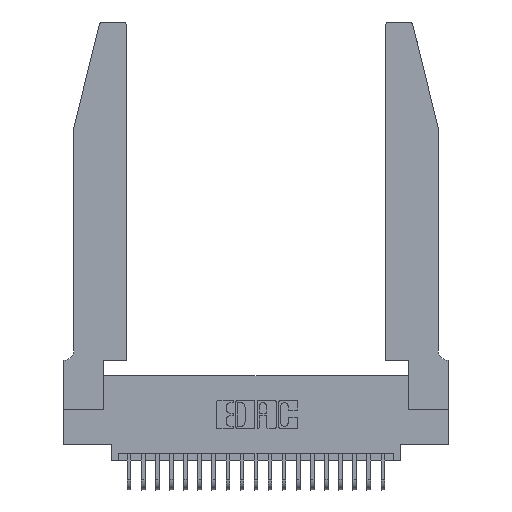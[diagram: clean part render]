
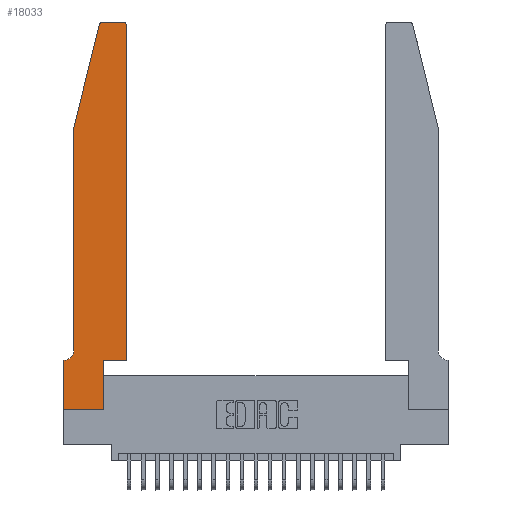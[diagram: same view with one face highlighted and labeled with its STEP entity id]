
A CAD part, top view. The second image highlights one B-rep face of the part: STEP entity #18033.
In plain terms, the highlighted planar face has unit normal (0, 0, 1).
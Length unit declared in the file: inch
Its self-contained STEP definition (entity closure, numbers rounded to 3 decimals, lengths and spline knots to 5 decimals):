
#156 = CARTESIAN_POINT ( 'NONE',  ( 0.2865, 0.35, 0.37 ) ) ;
#341 = DIRECTION ( 'NONE',  ( 0., 1., 0. ) ) ;
#700 = EDGE_CURVE ( 'NONE', #9601, #8523, #17865, .T. ) ;
#975 = AXIS2_PLACEMENT_3D ( 'NONE', #24388, #9488, #22736 ) ;
#1622 = ORIENTED_EDGE ( 'NONE', *, *, #17267, .T. ) ;
#1732 = VERTEX_POINT ( 'NONE', #7886 ) ;
#1825 = ORIENTED_EDGE ( 'NONE', *, *, #16543, .T. ) ;
#1904 = CARTESIAN_POINT ( 'NONE',  ( 0.0755, 2., 0.37 ) ) ;
#2159 = EDGE_CURVE ( 'NONE', #20746, #20488, #2907, .T. ) ;
#2433 = LINE ( 'NONE', #22900, #7492 ) ;
#2731 = VECTOR ( 'NONE', #8305, 39.37008 ) ;
#2771 = DIRECTION ( 'NONE',  ( 0., 0., 1. ) ) ;
#2834 = CARTESIAN_POINT ( 'NONE',  ( 0., 0.35, 0.37 ) ) ;
#2907 = LINE ( 'NONE', #1904, #13930 ) ;
#2929 = DIRECTION ( 'NONE',  ( 1., 0., 0. ) ) ;
#3110 = CARTESIAN_POINT ( 'NONE',  ( 0., 0.35, 0.37 ) ) ;
#3273 = CARTESIAN_POINT ( 'NONE',  ( 0.25487, 2.72718, 0.37 ) ) ;
#3785 = CARTESIAN_POINT ( 'NONE',  ( 0.284, 2.75, 0.37 ) ) ;
#4612 = ORIENTED_EDGE ( 'NONE', *, *, #8601, .T. ) ;
#4631 = EDGE_CURVE ( 'NONE', #8523, #17584, #9665, .T. ) ;
#4780 = DIRECTION ( 'NONE',  ( 0., 0., 1. ) ) ;
#4908 = DIRECTION ( 'NONE',  ( -1., 0., 0. ) ) ;
#5191 = ORIENTED_EDGE ( 'NONE', *, *, #14690, .T. ) ;
#5360 = CARTESIAN_POINT ( 'NONE',  ( 0.0055, 0.35, 0.37 ) ) ;
#5845 = ORIENTED_EDGE ( 'NONE', *, *, #16628, .T. ) ;
#6674 = LINE ( 'NONE', #6763, #18559 ) ;
#6763 = CARTESIAN_POINT ( 'NONE',  ( 0.0755, 0.35, 0.37 ) ) ;
#6802 = EDGE_CURVE ( 'NONE', #12399, #11351, #13110, .T. ) ;
#6941 = AXIS2_PLACEMENT_3D ( 'NONE', #19965, #2771, #2929 ) ;
#7134 = CARTESIAN_POINT ( 'NONE',  ( 0.2605, 2.75, 0.37 ) ) ;
#7492 = VECTOR ( 'NONE', #19033, 39.37008 ) ;
#7753 = LINE ( 'NONE', #22098, #22590 ) ;
#7847 = DIRECTION ( 'NONE',  ( -1., 0., 0. ) ) ;
#7886 = CARTESIAN_POINT ( 'NONE',  ( 0.4505, 0.35, 0.37 ) ) ;
#8224 = CIRCLE ( 'NONE', #14973, 0.07 ) ;
#8305 = DIRECTION ( 'NONE',  ( 0., -1., 0. ) ) ;
#8496 = LINE ( 'NONE', #12520, #22703 ) ;
#8523 = VERTEX_POINT ( 'NONE', #23168 ) ;
#8601 = EDGE_CURVE ( 'NONE', #14361, #12399, #6674, .T. ) ;
#8809 = VECTOR ( 'NONE', #20412, 39.37008 ) ;
#9139 = ORIENTED_EDGE ( 'NONE', *, *, #23587, .T. ) ;
#9287 = VERTEX_POINT ( 'NONE', #3273 ) ;
#9488 = DIRECTION ( 'NONE',  ( 0., 0., 1. ) ) ;
#9601 = VERTEX_POINT ( 'NONE', #24512 ) ;
#9665 = LINE ( 'NONE', #7134, #8809 ) ;
#10424 = ORIENTED_EDGE ( 'NONE', *, *, #12999, .T. ) ;
#10481 = EDGE_CURVE ( 'NONE', #11351, #22483, #7753, .T. ) ;
#10735 = DIRECTION ( 'NONE',  ( 1., 0., 0. ) ) ;
#11276 = VECTOR ( 'NONE', #18598, 39.37008 ) ;
#11351 = VERTEX_POINT ( 'NONE', #12797 ) ;
#12108 = ORIENTED_EDGE ( 'NONE', *, *, #700, .T. ) ;
#12293 = CARTESIAN_POINT ( 'NONE',  ( 0.4505, 0.35, 0.37 ) ) ;
#12399 = VERTEX_POINT ( 'NONE', #2834 ) ;
#12520 = CARTESIAN_POINT ( 'NONE',  ( 0.4505, 0.35, 0.37 ) ) ;
#12797 = CARTESIAN_POINT ( 'NONE',  ( 0., 0., 0.37 ) ) ;
#12999 = EDGE_CURVE ( 'NONE', #20488, #14361, #8224, .T. ) ;
#13086 = FACE_OUTER_BOUND ( 'NONE', #18027, .T. ) ;
#13110 = LINE ( 'NONE', #23144, #2731 ) ;
#13841 = ORIENTED_EDGE ( 'NONE', *, *, #6802, .T. ) ;
#13930 = VECTOR ( 'NONE', #15843, 39.37008 ) ;
#14361 = VERTEX_POINT ( 'NONE', #5360 ) ;
#14690 = EDGE_CURVE ( 'NONE', #1732, #9601, #8496, .T. ) ;
#14915 = ORIENTED_EDGE ( 'NONE', *, *, #2159, .T. ) ;
#14973 = AXIS2_PLACEMENT_3D ( 'NONE', #22853, #19228, #7847 ) ;
#15843 = DIRECTION ( 'NONE',  ( 0., -1., 0. ) ) ;
#16248 = DIRECTION ( 'NONE',  ( 1., 0., 0. ) ) ;
#16349 = LINE ( 'NONE', #12293, #11276 ) ;
#16543 = EDGE_CURVE ( 'NONE', #17584, #9287, #18203, .T. ) ;
#16628 = EDGE_CURVE ( 'NONE', #9287, #20746, #2433, .T. ) ;
#16680 = LINE ( 'NONE', #156, #16967 ) ;
#16967 = VECTOR ( 'NONE', #341, 39.37008 ) ;
#17267 = EDGE_CURVE ( 'NONE', #22483, #20730, #16680, .T. ) ;
#17395 = CARTESIAN_POINT ( 'NONE',  ( 0.2865, 0.35, 0.37 ) ) ;
#17584 = VERTEX_POINT ( 'NONE', #3785 ) ;
#17865 = CIRCLE ( 'NONE', #6941, 0.03 ) ;
#18027 = EDGE_LOOP ( 'NONE', ( #19809, #1825, #5845, #14915, #10424, #4612, #13841, #20931, #1622, #9139, #5191, #12108 ) ) ;
#18033 = ADVANCED_FACE ( 'NONE', ( #13086 ), #21810, .T. ) ;
#18178 = DIRECTION ( 'NONE',  ( 0., 1., 0. ) ) ;
#18203 = CIRCLE ( 'NONE', #975, 0.03 ) ;
#18559 = VECTOR ( 'NONE', #4908, 39.37008 ) ;
#18598 = DIRECTION ( 'NONE',  ( 1., 0., 0. ) ) ;
#18737 = CARTESIAN_POINT ( 'NONE',  ( 0.0755, 0.42, 0.37 ) ) ;
#19033 = DIRECTION ( 'NONE',  ( -0.239, -0.971, 0. ) ) ;
#19228 = DIRECTION ( 'NONE',  ( 0., 0., -1. ) ) ;
#19405 = CARTESIAN_POINT ( 'NONE',  ( 0.2865, 0., 0.37 ) ) ;
#19809 = ORIENTED_EDGE ( 'NONE', *, *, #4631, .T. ) ;
#19965 = CARTESIAN_POINT ( 'NONE',  ( 0.4205, 2.72, 0.37 ) ) ;
#20412 = DIRECTION ( 'NONE',  ( -1., 0., 0. ) ) ;
#20488 = VERTEX_POINT ( 'NONE', #18737 ) ;
#20730 = VERTEX_POINT ( 'NONE', #17395 ) ;
#20746 = VERTEX_POINT ( 'NONE', #22780 ) ;
#20931 = ORIENTED_EDGE ( 'NONE', *, *, #10481, .T. ) ;
#21810 = PLANE ( 'NONE',  #23838 ) ;
#22098 = CARTESIAN_POINT ( 'NONE',  ( 0., 0., 0.37 ) ) ;
#22483 = VERTEX_POINT ( 'NONE', #19405 ) ;
#22590 = VECTOR ( 'NONE', #10735, 39.37008 ) ;
#22703 = VECTOR ( 'NONE', #18178, 39.37008 ) ;
#22736 = DIRECTION ( 'NONE',  ( 1., 0., 0. ) ) ;
#22780 = CARTESIAN_POINT ( 'NONE',  ( 0.0755, 2., 0.37 ) ) ;
#22853 = CARTESIAN_POINT ( 'NONE',  ( 0.0055, 0.42, 0.37 ) ) ;
#22900 = CARTESIAN_POINT ( 'NONE',  ( 0.0755, 2., 0.37 ) ) ;
#23144 = CARTESIAN_POINT ( 'NONE',  ( 0., 0., 0.37 ) ) ;
#23168 = CARTESIAN_POINT ( 'NONE',  ( 0.4205, 2.75, 0.37 ) ) ;
#23587 = EDGE_CURVE ( 'NONE', #20730, #1732, #16349, .T. ) ;
#23838 = AXIS2_PLACEMENT_3D ( 'NONE', #3110, #4780, #16248 ) ;
#24388 = CARTESIAN_POINT ( 'NONE',  ( 0.284, 2.72, 0.37 ) ) ;
#24512 = CARTESIAN_POINT ( 'NONE',  ( 0.4505, 2.72, 0.37 ) ) ;
